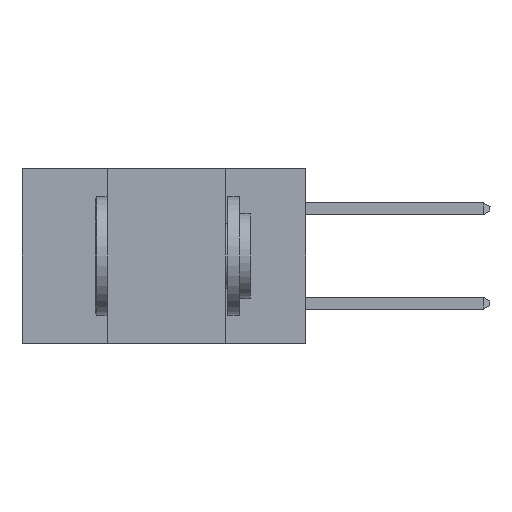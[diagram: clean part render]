
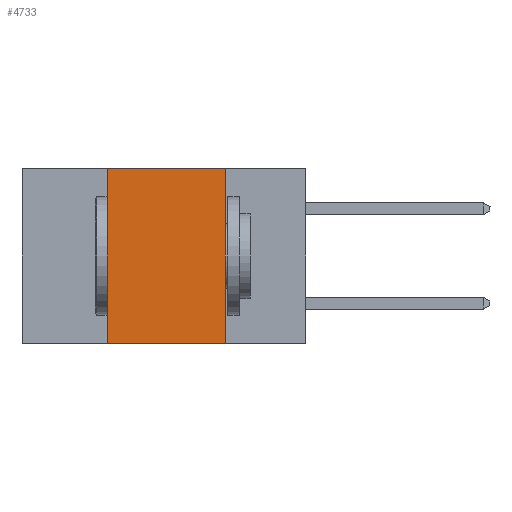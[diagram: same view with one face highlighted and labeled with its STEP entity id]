
A CAD part, left-side view. The second image highlights one B-rep face of the part: STEP entity #4733.
In plain terms, the highlighted planar face has unit normal (-1, 0, 0).
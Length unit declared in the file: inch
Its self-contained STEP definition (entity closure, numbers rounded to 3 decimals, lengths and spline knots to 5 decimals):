
#559 = EDGE_LOOP ( 'NONE', ( #7177, #15663, #7279, #8598 ) ) ;
#578 = CARTESIAN_POINT ( 'NONE',  ( 0., 0.6, 0. ) ) ;
#1258 = DIRECTION ( 'NONE',  ( 0., -1., 0. ) ) ;
#1856 = CARTESIAN_POINT ( 'NONE',  ( 0., 0.6, 0. ) ) ;
#2177 = VECTOR ( 'NONE', #18575, 39.37008 ) ;
#3188 = LINE ( 'NONE', #3786, #17523 ) ;
#3786 = CARTESIAN_POINT ( 'NONE',  ( 0., 0.42, 0. ) ) ;
#3877 = DIRECTION ( 'NONE',  ( 0., 0., -1. ) ) ;
#4733 = ADVANCED_FACE ( 'NONE', ( #13837 ), #12258, .F. ) ;
#5845 = AXIS2_PLACEMENT_3D ( 'NONE', #578, #16962, #3877 ) ;
#6009 = VECTOR ( 'NONE', #16612, 39.37008 ) ;
#6336 = CARTESIAN_POINT ( 'NONE',  ( 0., 0.42, 0. ) ) ;
#7042 = CARTESIAN_POINT ( 'NONE',  ( 0., 0.17, -0.37 ) ) ;
#7177 = ORIENTED_EDGE ( 'NONE', *, *, #10037, .F. ) ;
#7279 = ORIENTED_EDGE ( 'NONE', *, *, #18498, .F. ) ;
#8598 = ORIENTED_EDGE ( 'NONE', *, *, #10904, .T. ) ;
#8950 = VERTEX_POINT ( 'NONE', #15159 ) ;
#10037 = EDGE_CURVE ( 'NONE', #8950, #18503, #16292, .T. ) ;
#10904 = EDGE_CURVE ( 'NONE', #13068, #18503, #12918, .T. ) ;
#11227 = CARTESIAN_POINT ( 'NONE',  ( 0., 0.6, -0.37 ) ) ;
#12037 = DIRECTION ( 'NONE',  ( 0., 0., 1. ) ) ;
#12258 = PLANE ( 'NONE',  #5845 ) ;
#12918 = LINE ( 'NONE', #11227, #16227 ) ;
#13068 = VERTEX_POINT ( 'NONE', #21049 ) ;
#13837 = FACE_OUTER_BOUND ( 'NONE', #559, .T. ) ;
#15159 = CARTESIAN_POINT ( 'NONE',  ( 0., 0.17, 0. ) ) ;
#15663 = ORIENTED_EDGE ( 'NONE', *, *, #17170, .F. ) ;
#16227 = VECTOR ( 'NONE', #1258, 39.37008 ) ;
#16292 = LINE ( 'NONE', #18518, #2177 ) ;
#16612 = DIRECTION ( 'NONE',  ( 0., -1., 0. ) ) ;
#16870 = VERTEX_POINT ( 'NONE', #6336 ) ;
#16962 = DIRECTION ( 'NONE',  ( 1., 0., 0. ) ) ;
#17170 = EDGE_CURVE ( 'NONE', #16870, #8950, #18287, .T. ) ;
#17523 = VECTOR ( 'NONE', #12037, 39.37008 ) ;
#18287 = LINE ( 'NONE', #1856, #6009 ) ;
#18498 = EDGE_CURVE ( 'NONE', #13068, #16870, #3188, .T. ) ;
#18503 = VERTEX_POINT ( 'NONE', #7042 ) ;
#18518 = CARTESIAN_POINT ( 'NONE',  ( 0., 0.17, 0. ) ) ;
#18575 = DIRECTION ( 'NONE',  ( 0., 0., -1. ) ) ;
#21049 = CARTESIAN_POINT ( 'NONE',  ( 0., 0.42, -0.37 ) ) ;
